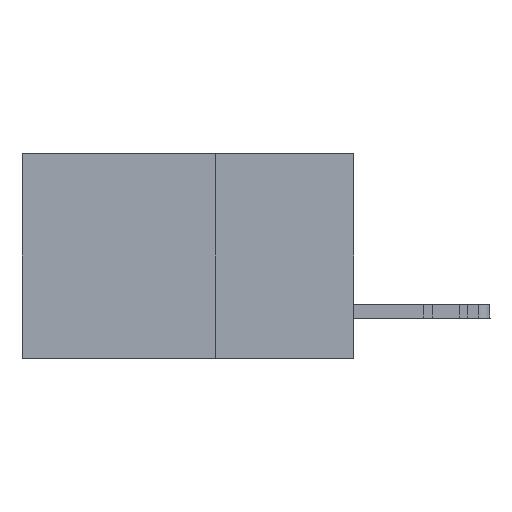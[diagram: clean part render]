
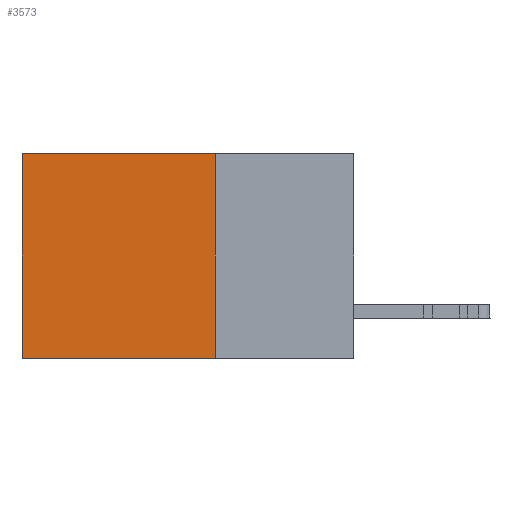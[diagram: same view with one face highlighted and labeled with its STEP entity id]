
A CAD part, left-side view. The second image highlights one B-rep face of the part: STEP entity #3573.
In plain terms, the highlighted planar face has unit normal (-1, 0, 0).
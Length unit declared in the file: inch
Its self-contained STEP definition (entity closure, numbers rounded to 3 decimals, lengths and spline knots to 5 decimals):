
#900 = ORIENTED_EDGE ( 'NONE', *, *, #28283, .T. ) ;
#2617 = VERTEX_POINT ( 'NONE', #23343 ) ;
#2731 = DIRECTION ( 'NONE',  ( 0., 0., -1. ) ) ;
#3039 = VERTEX_POINT ( 'NONE', #20302 ) ;
#3573 = ADVANCED_FACE ( 'NONE', ( #46713 ), #38305, .F. ) ;
#4690 = ORIENTED_EDGE ( 'NONE', *, *, #18751, .T. ) ;
#10121 = CARTESIAN_POINT ( 'NONE',  ( 0.2875, 0.25, -0.37 ) ) ;
#10428 = CARTESIAN_POINT ( 'NONE',  ( 0.2875, 0.6, 0. ) ) ;
#12366 = CARTESIAN_POINT ( 'NONE',  ( 0.2875, 0.25, 0. ) ) ;
#14192 = LINE ( 'NONE', #18149, #42522 ) ;
#15455 = CARTESIAN_POINT ( 'NONE',  ( 0.2875, 0.6, -0.37 ) ) ;
#16582 = VECTOR ( 'NONE', #18990, 39.37008 ) ;
#17623 = ORIENTED_EDGE ( 'NONE', *, *, #26580, .F. ) ;
#18149 = CARTESIAN_POINT ( 'NONE',  ( 0.2875, 0.6, 0. ) ) ;
#18290 = AXIS2_PLACEMENT_3D ( 'NONE', #21351, #20717, #2731 ) ;
#18751 = EDGE_CURVE ( 'NONE', #25951, #29978, #14192, .T. ) ;
#18990 = DIRECTION ( 'NONE',  ( 0., 0., -1. ) ) ;
#19478 = CARTESIAN_POINT ( 'NONE',  ( 0.2875, 0.25, 0. ) ) ;
#20302 = CARTESIAN_POINT ( 'NONE',  ( 0.2875, 0.25, -0.37 ) ) ;
#20586 = VECTOR ( 'NONE', #46401, 39.37008 ) ;
#20717 = DIRECTION ( 'NONE',  ( 1., 0., 0. ) ) ;
#21351 = CARTESIAN_POINT ( 'NONE',  ( 0.2875, 0.25, 0. ) ) ;
#22674 = LINE ( 'NONE', #19478, #31173 ) ;
#23343 = CARTESIAN_POINT ( 'NONE',  ( 0.2875, 0.25, 0. ) ) ;
#23433 = LINE ( 'NONE', #12366, #16582 ) ;
#25951 = VERTEX_POINT ( 'NONE', #10428 ) ;
#26580 = EDGE_CURVE ( 'NONE', #3039, #29978, #29597, .T. ) ;
#28283 = EDGE_CURVE ( 'NONE', #2617, #25951, #22674, .T. ) ;
#29597 = LINE ( 'NONE', #10121, #20586 ) ;
#29978 = VERTEX_POINT ( 'NONE', #15455 ) ;
#31173 = VECTOR ( 'NONE', #45010, 39.37008 ) ;
#37546 = EDGE_LOOP ( 'NONE', ( #4690, #17623, #43897, #900 ) ) ;
#38305 = PLANE ( 'NONE',  #18290 ) ;
#38657 = EDGE_CURVE ( 'NONE', #2617, #3039, #23433, .T. ) ;
#40818 = DIRECTION ( 'NONE',  ( 0., 0., -1. ) ) ;
#42522 = VECTOR ( 'NONE', #40818, 39.37008 ) ;
#43897 = ORIENTED_EDGE ( 'NONE', *, *, #38657, .F. ) ;
#45010 = DIRECTION ( 'NONE',  ( 0., 1., 0. ) ) ;
#46401 = DIRECTION ( 'NONE',  ( 0., 1., 0. ) ) ;
#46713 = FACE_OUTER_BOUND ( 'NONE', #37546, .T. ) ;
